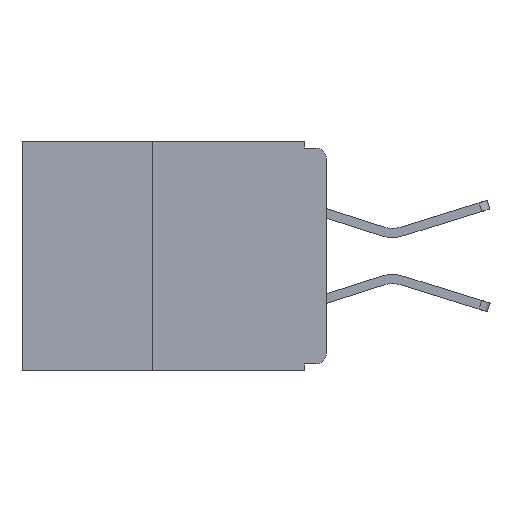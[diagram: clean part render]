
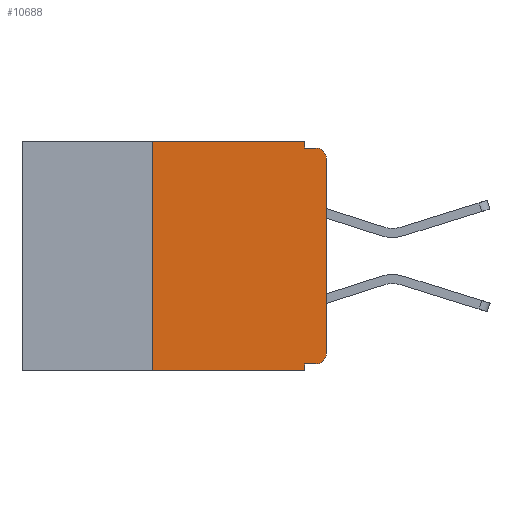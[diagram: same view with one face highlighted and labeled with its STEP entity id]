
A CAD part, left-side view. The second image highlights one B-rep face of the part: STEP entity #10688.
In plain terms, the highlighted planar face has unit normal (-1, 0, 0).
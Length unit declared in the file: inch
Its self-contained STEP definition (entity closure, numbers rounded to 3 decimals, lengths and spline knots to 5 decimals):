
#59 = VECTOR ( 'NONE', #12748, 39.37008 ) ;
#623 = DIRECTION ( 'NONE',  ( 1., 0., 0. ) ) ;
#814 = DIRECTION ( 'NONE',  ( 0., 0., -1. ) ) ;
#853 = DIRECTION ( 'NONE',  ( -1., 0., 0. ) ) ;
#855 = CARTESIAN_POINT ( 'NONE',  ( 0., 0.015, -0.305 ) ) ;
#981 = VERTEX_POINT ( 'NONE', #8859 ) ;
#1335 = EDGE_CURVE ( 'NONE', #14781, #15840, #8315, .T. ) ;
#1735 = DIRECTION ( 'NONE',  ( 0., 0., 1. ) ) ;
#1834 = CARTESIAN_POINT ( 'NONE',  ( 0., 0.031, -0.32 ) ) ;
#1908 = LINE ( 'NONE', #17220, #7179 ) ;
#2066 = VERTEX_POINT ( 'NONE', #4734 ) ;
#2257 = ORIENTED_EDGE ( 'NONE', *, *, #10784, .T. ) ;
#2284 = DIRECTION ( 'NONE',  ( -1., 0., 0. ) ) ;
#2562 = AXIS2_PLACEMENT_3D ( 'NONE', #18000, #623, #10843 ) ;
#2583 = DIRECTION ( 'NONE',  ( 0., 0., 1. ) ) ;
#2645 = CARTESIAN_POINT ( 'NONE',  ( 0., 0.25, -0.33 ) ) ;
#2985 = CIRCLE ( 'NONE', #5539, 0.015 ) ;
#3112 = DIRECTION ( 'NONE',  ( 0., -1., 0. ) ) ;
#3249 = ORIENTED_EDGE ( 'NONE', *, *, #1335, .F. ) ;
#3286 = VERTEX_POINT ( 'NONE', #17898 ) ;
#3399 = CARTESIAN_POINT ( 'NONE',  ( 0., 0., -0.01 ) ) ;
#4450 = LINE ( 'NONE', #14293, #11692 ) ;
#4622 = EDGE_CURVE ( 'NONE', #14781, #10555, #6606, .T. ) ;
#4734 = CARTESIAN_POINT ( 'NONE',  ( 0., 0.031, -0.01 ) ) ;
#5083 = DIRECTION ( 'NONE',  ( 0., 0., -1. ) ) ;
#5539 = AXIS2_PLACEMENT_3D ( 'NONE', #11019, #2284, #12492 ) ;
#5907 = LINE ( 'NONE', #8060, #16981 ) ;
#6327 = VERTEX_POINT ( 'NONE', #10756 ) ;
#6606 = CIRCLE ( 'NONE', #15418, 0.015 ) ;
#7162 = VECTOR ( 'NONE', #14064, 39.37008 ) ;
#7179 = VECTOR ( 'NONE', #17262, 39.37008 ) ;
#7647 = EDGE_CURVE ( 'NONE', #10885, #2066, #1908, .T. ) ;
#8006 = ORIENTED_EDGE ( 'NONE', *, *, #7647, .F. ) ;
#8060 = CARTESIAN_POINT ( 'NONE',  ( 0., 0.437, 0. ) ) ;
#8118 = EDGE_CURVE ( 'NONE', #2066, #981, #13074, .T. ) ;
#8165 = EDGE_CURVE ( 'NONE', #18069, #3286, #9664, .T. ) ;
#8308 = VERTEX_POINT ( 'NONE', #17833 ) ;
#8315 = LINE ( 'NONE', #13464, #59 ) ;
#8452 = ORIENTED_EDGE ( 'NONE', *, *, #17812, .F. ) ;
#8616 = CARTESIAN_POINT ( 'NONE',  ( 0., 0.25, -0.33 ) ) ;
#8646 = EDGE_CURVE ( 'NONE', #18069, #6327, #11939, .T. ) ;
#8710 = ORIENTED_EDGE ( 'NONE', *, *, #8165, .F. ) ;
#8859 = CARTESIAN_POINT ( 'NONE',  ( 0., 0.015, -0.01 ) ) ;
#9508 = DIRECTION ( 'NONE',  ( 0., -1., 0. ) ) ;
#9622 = ORIENTED_EDGE ( 'NONE', *, *, #10721, .F. ) ;
#9664 = LINE ( 'NONE', #2645, #12157 ) ;
#10555 = VERTEX_POINT ( 'NONE', #16334 ) ;
#10688 = ADVANCED_FACE ( 'NONE', ( #11628 ), #17937, .F. ) ;
#10721 = EDGE_CURVE ( 'NONE', #15840, #6327, #11180, .T. ) ;
#10756 = CARTESIAN_POINT ( 'NONE',  ( 0., 0.031, -0.33 ) ) ;
#10784 = EDGE_CURVE ( 'NONE', #8308, #981, #2985, .T. ) ;
#10843 = DIRECTION ( 'NONE',  ( 0., 0., -1. ) ) ;
#10885 = VERTEX_POINT ( 'NONE', #11283 ) ;
#10908 = CARTESIAN_POINT ( 'NONE',  ( 0., 0.031, -0.33 ) ) ;
#11019 = CARTESIAN_POINT ( 'NONE',  ( 0., 0.015, -0.025 ) ) ;
#11180 = LINE ( 'NONE', #10908, #18361 ) ;
#11283 = CARTESIAN_POINT ( 'NONE',  ( 0., 0.031, 0. ) ) ;
#11628 = FACE_OUTER_BOUND ( 'NONE', #15658, .T. ) ;
#11692 = VECTOR ( 'NONE', #2583, 39.37008 ) ;
#11939 = LINE ( 'NONE', #14199, #7162 ) ;
#12157 = VECTOR ( 'NONE', #1735, 39.37008 ) ;
#12492 = DIRECTION ( 'NONE',  ( 0., 0., -1. ) ) ;
#12748 = DIRECTION ( 'NONE',  ( 0., 1., 0. ) ) ;
#13074 = LINE ( 'NONE', #3399, #13991 ) ;
#13464 = CARTESIAN_POINT ( 'NONE',  ( 0., 0., -0.32 ) ) ;
#13513 = CARTESIAN_POINT ( 'NONE',  ( 0., 0.015, -0.32 ) ) ;
#13861 = EDGE_CURVE ( 'NONE', #10555, #8308, #4450, .T. ) ;
#13991 = VECTOR ( 'NONE', #3112, 39.37008 ) ;
#14064 = DIRECTION ( 'NONE',  ( 0., -1., 0. ) ) ;
#14199 = CARTESIAN_POINT ( 'NONE',  ( 0., 0.437, -0.33 ) ) ;
#14293 = CARTESIAN_POINT ( 'NONE',  ( 0., 0., 0. ) ) ;
#14781 = VERTEX_POINT ( 'NONE', #13513 ) ;
#15418 = AXIS2_PLACEMENT_3D ( 'NONE', #855, #853, #814 ) ;
#15658 = EDGE_LOOP ( 'NONE', ( #17223, #2257, #18131, #8006, #8452, #8710, #16833, #9622, #3249, #15753 ) ) ;
#15753 = ORIENTED_EDGE ( 'NONE', *, *, #4622, .T. ) ;
#15840 = VERTEX_POINT ( 'NONE', #1834 ) ;
#16334 = CARTESIAN_POINT ( 'NONE',  ( 0., 0., -0.305 ) ) ;
#16833 = ORIENTED_EDGE ( 'NONE', *, *, #8646, .T. ) ;
#16981 = VECTOR ( 'NONE', #9508, 39.37008 ) ;
#17220 = CARTESIAN_POINT ( 'NONE',  ( 0., 0.031, 0. ) ) ;
#17223 = ORIENTED_EDGE ( 'NONE', *, *, #13861, .T. ) ;
#17262 = DIRECTION ( 'NONE',  ( 0., 0., -1. ) ) ;
#17812 = EDGE_CURVE ( 'NONE', #3286, #10885, #5907, .T. ) ;
#17833 = CARTESIAN_POINT ( 'NONE',  ( 0., 0., -0.025 ) ) ;
#17898 = CARTESIAN_POINT ( 'NONE',  ( 0., 0.25, 0. ) ) ;
#17937 = PLANE ( 'NONE',  #2562 ) ;
#18000 = CARTESIAN_POINT ( 'NONE',  ( 0., 0.437, 0. ) ) ;
#18069 = VERTEX_POINT ( 'NONE', #8616 ) ;
#18131 = ORIENTED_EDGE ( 'NONE', *, *, #8118, .F. ) ;
#18361 = VECTOR ( 'NONE', #5083, 39.37008 ) ;
